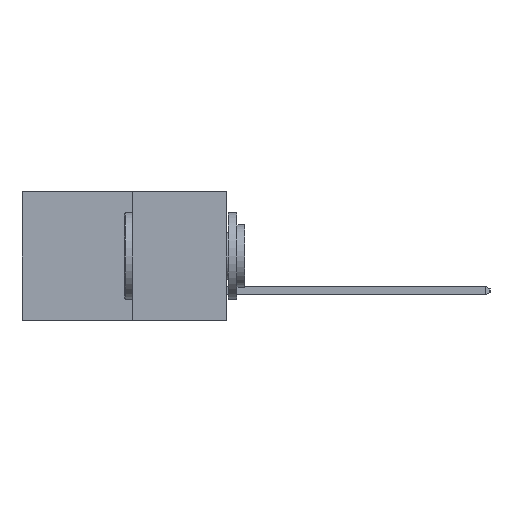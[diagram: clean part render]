
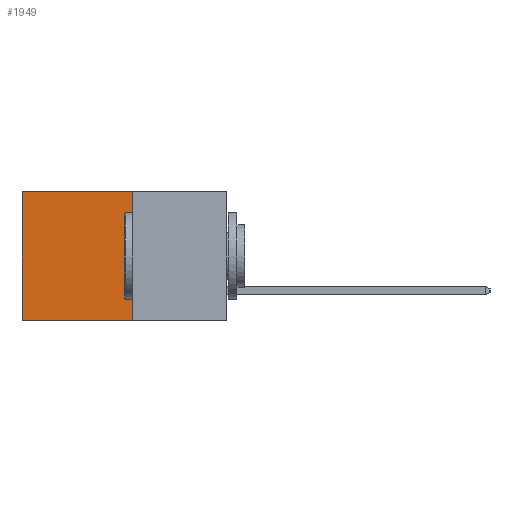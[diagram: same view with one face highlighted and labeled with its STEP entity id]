
A CAD part, left-side view. The second image highlights one B-rep face of the part: STEP entity #1949.
In plain terms, the highlighted planar face has unit normal (-1, 0, 0).
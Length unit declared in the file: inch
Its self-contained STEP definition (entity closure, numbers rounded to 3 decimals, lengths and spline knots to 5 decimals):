
#50 = LINE ( 'NONE', #13616, #9244 ) ;
#109 = ORIENTED_EDGE ( 'NONE', *, *, #2887, .F. ) ;
#393 = VECTOR ( 'NONE', #8124, 39.37008 ) ;
#612 = AXIS2_PLACEMENT_3D ( 'NONE', #6951, #1916, #1934 ) ;
#949 = CARTESIAN_POINT ( 'NONE',  ( 0.277, 0.59, 0. ) ) ;
#1077 = EDGE_LOOP ( 'NONE', ( #3311, #8555, #109, #2988 ) ) ;
#1550 = FACE_OUTER_BOUND ( 'NONE', #1077, .T. ) ;
#1754 = VERTEX_POINT ( 'NONE', #5346 ) ;
#1916 = DIRECTION ( 'NONE',  ( 1., 0., 0. ) ) ;
#1934 = DIRECTION ( 'NONE',  ( 0., 0., -1. ) ) ;
#1949 = ADVANCED_FACE ( 'NONE', ( #1550 ), #6393, .F. ) ;
#1983 = CARTESIAN_POINT ( 'NONE',  ( 0.277, 0.27, -0.37 ) ) ;
#2752 = CARTESIAN_POINT ( 'NONE',  ( 0.277, 0.27, 0. ) ) ;
#2887 = EDGE_CURVE ( 'NONE', #1754, #13947, #6548, .T. ) ;
#2988 = ORIENTED_EDGE ( 'NONE', *, *, #9131, .T. ) ;
#3311 = ORIENTED_EDGE ( 'NONE', *, *, #6961, .T. ) ;
#4705 = DIRECTION ( 'NONE',  ( 0., 0., -1. ) ) ;
#5346 = CARTESIAN_POINT ( 'NONE',  ( 0.277, 0.27, 0. ) ) ;
#6125 = LINE ( 'NONE', #10368, #393 ) ;
#6393 = PLANE ( 'NONE',  #612 ) ;
#6548 = LINE ( 'NONE', #9632, #12598 ) ;
#6951 = CARTESIAN_POINT ( 'NONE',  ( 0.277, 0.27, -0.37 ) ) ;
#6961 = EDGE_CURVE ( 'NONE', #14548, #10519, #50, .T. ) ;
#8124 = DIRECTION ( 'NONE',  ( 0., 1., 0. ) ) ;
#8555 = ORIENTED_EDGE ( 'NONE', *, *, #11385, .F. ) ;
#8744 = CARTESIAN_POINT ( 'NONE',  ( 0.277, 0.59, -0.37 ) ) ;
#9131 = EDGE_CURVE ( 'NONE', #1754, #14548, #9865, .T. ) ;
#9244 = VECTOR ( 'NONE', #13774, 39.37008 ) ;
#9632 = CARTESIAN_POINT ( 'NONE',  ( 0.277, 0.27, -0.37 ) ) ;
#9865 = LINE ( 'NONE', #2752, #12493 ) ;
#10368 = CARTESIAN_POINT ( 'NONE',  ( 0.277, 0.27, -0.37 ) ) ;
#10519 = VERTEX_POINT ( 'NONE', #8744 ) ;
#11385 = EDGE_CURVE ( 'NONE', #13947, #10519, #6125, .T. ) ;
#12493 = VECTOR ( 'NONE', #13021, 39.37008 ) ;
#12598 = VECTOR ( 'NONE', #4705, 39.37008 ) ;
#13021 = DIRECTION ( 'NONE',  ( 0., 1., 0. ) ) ;
#13616 = CARTESIAN_POINT ( 'NONE',  ( 0.277, 0.59, -0.37 ) ) ;
#13774 = DIRECTION ( 'NONE',  ( 0., 0., -1. ) ) ;
#13947 = VERTEX_POINT ( 'NONE', #1983 ) ;
#14548 = VERTEX_POINT ( 'NONE', #949 ) ;
